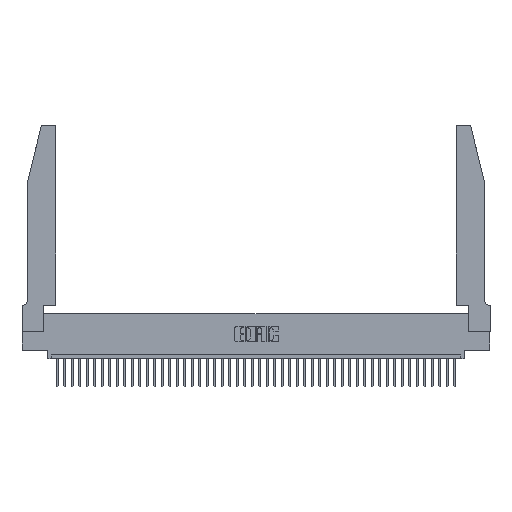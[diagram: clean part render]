
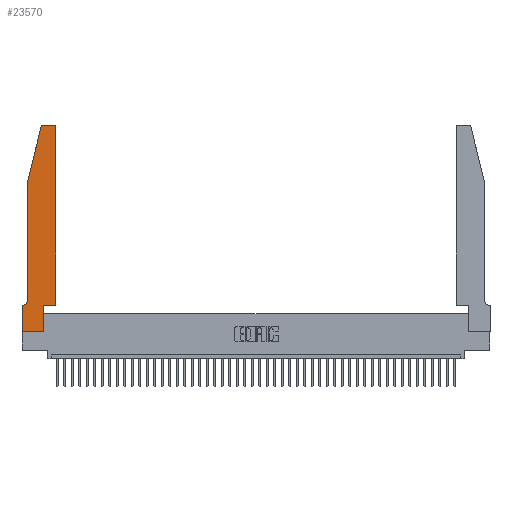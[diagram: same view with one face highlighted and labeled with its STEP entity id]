
A CAD part, top view. The second image highlights one B-rep face of the part: STEP entity #23570.
In plain terms, the highlighted planar face has unit normal (0, 0, 1).
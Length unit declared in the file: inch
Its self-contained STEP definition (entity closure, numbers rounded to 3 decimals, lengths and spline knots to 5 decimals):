
#668 = AXIS2_PLACEMENT_3D ( 'NONE', #10846, #24647, #20948 ) ;
#816 = CARTESIAN_POINT ( 'NONE',  ( 0.0755, 2., 0.37 ) ) ;
#941 = DIRECTION ( 'NONE',  ( -1., 0., 0. ) ) ;
#1044 = CIRCLE ( 'NONE', #10132, 0.03 ) ;
#1135 = CARTESIAN_POINT ( 'NONE',  ( 0.2865, 0.35, 0.37 ) ) ;
#1414 = VERTEX_POINT ( 'NONE', #2004 ) ;
#2004 = CARTESIAN_POINT ( 'NONE',  ( 0.4505, 0.35, 0.37 ) ) ;
#2997 = EDGE_CURVE ( 'NONE', #4055, #8257, #1044, .T. ) ;
#4055 = VERTEX_POINT ( 'NONE', #32065 ) ;
#4761 = ORIENTED_EDGE ( 'NONE', *, *, #34002, .T. ) ;
#5108 = EDGE_CURVE ( 'NONE', #13053, #29665, #31711, .T. ) ;
#5269 = DIRECTION ( 'NONE',  ( 0., 1., 0. ) ) ;
#5386 = EDGE_CURVE ( 'NONE', #9681, #40438, #21077, .T. ) ;
#5597 = DIRECTION ( 'NONE',  ( 1., 0., 0. ) ) ;
#7216 = ORIENTED_EDGE ( 'NONE', *, *, #5108, .T. ) ;
#7484 = CARTESIAN_POINT ( 'NONE',  ( 0., 0., 0.37 ) ) ;
#8257 = VERTEX_POINT ( 'NONE', #11931 ) ;
#8695 = CARTESIAN_POINT ( 'NONE',  ( 0., 0., 0.37 ) ) ;
#9653 = DIRECTION ( 'NONE',  ( 1., 0., 0. ) ) ;
#9681 = VERTEX_POINT ( 'NONE', #16517 ) ;
#10132 = AXIS2_PLACEMENT_3D ( 'NONE', #18822, #42362, #22064 ) ;
#10153 = DIRECTION ( 'NONE',  ( -0.239, -0.971, 0. ) ) ;
#10846 = CARTESIAN_POINT ( 'NONE',  ( 0.284, 2.72, 0.37 ) ) ;
#11004 = LINE ( 'NONE', #19722, #29632 ) ;
#11197 = CARTESIAN_POINT ( 'NONE',  ( 0.0755, 0.35, 0.37 ) ) ;
#11525 = VECTOR ( 'NONE', #5269, 39.37008 ) ;
#11547 = CARTESIAN_POINT ( 'NONE',  ( 0., 0.35, 0.37 ) ) ;
#11931 = CARTESIAN_POINT ( 'NONE',  ( 0.4205, 2.75, 0.37 ) ) ;
#12496 = VECTOR ( 'NONE', #18956, 39.37008 ) ;
#13053 = VERTEX_POINT ( 'NONE', #22299 ) ;
#13202 = VECTOR ( 'NONE', #10153, 39.37008 ) ;
#13825 = CARTESIAN_POINT ( 'NONE',  ( 0.0755, 0.42, 0.37 ) ) ;
#14412 = VECTOR ( 'NONE', #5597, 39.37008 ) ;
#14427 = VERTEX_POINT ( 'NONE', #13825 ) ;
#15261 = CARTESIAN_POINT ( 'NONE',  ( 0.0755, 2., 0.37 ) ) ;
#15931 = VECTOR ( 'NONE', #38326, 39.37008 ) ;
#16517 = CARTESIAN_POINT ( 'NONE',  ( 0.2865, 0., 0.37 ) ) ;
#18342 = ORIENTED_EDGE ( 'NONE', *, *, #22593, .T. ) ;
#18578 = LINE ( 'NONE', #33830, #21210 ) ;
#18591 = CARTESIAN_POINT ( 'NONE',  ( 0., 0.35, 0.37 ) ) ;
#18822 = CARTESIAN_POINT ( 'NONE',  ( 0.4205, 2.72, 0.37 ) ) ;
#18956 = DIRECTION ( 'NONE',  ( -1., 0., 0. ) ) ;
#19722 = CARTESIAN_POINT ( 'NONE',  ( 0.4505, 0.35, 0.37 ) ) ;
#19889 = EDGE_LOOP ( 'NONE', ( #4761, #30393, #7216, #40373, #22194, #21090, #22192, #24169, #32950, #18342, #26934, #23858 ) ) ;
#20124 = FACE_OUTER_BOUND ( 'NONE', #19889, .T. ) ;
#20133 = VERTEX_POINT ( 'NONE', #21171 ) ;
#20267 = CARTESIAN_POINT ( 'NONE',  ( 0.0755, 2., 0.37 ) ) ;
#20818 = AXIS2_PLACEMENT_3D ( 'NONE', #11547, #24437, #38428 ) ;
#20943 = CARTESIAN_POINT ( 'NONE',  ( 0.284, 2.75, 0.37 ) ) ;
#20948 = DIRECTION ( 'NONE',  ( 1., 0., 0. ) ) ;
#21077 = LINE ( 'NONE', #31662, #11525 ) ;
#21090 = ORIENTED_EDGE ( 'NONE', *, *, #36607, .T. ) ;
#21168 = CARTESIAN_POINT ( 'NONE',  ( 0.0055, 0.42, 0.37 ) ) ;
#21171 = CARTESIAN_POINT ( 'NONE',  ( 0., 0., 0.37 ) ) ;
#21177 = EDGE_CURVE ( 'NONE', #20133, #9681, #29898, .T. ) ;
#21210 = VECTOR ( 'NONE', #9653, 39.37008 ) ;
#21493 = LINE ( 'NONE', #42050, #12496 ) ;
#21993 = VECTOR ( 'NONE', #34496, 39.37008 ) ;
#22064 = DIRECTION ( 'NONE',  ( 1., 0., 0. ) ) ;
#22192 = ORIENTED_EDGE ( 'NONE', *, *, #25348, .T. ) ;
#22194 = ORIENTED_EDGE ( 'NONE', *, *, #41020, .T. ) ;
#22299 = CARTESIAN_POINT ( 'NONE',  ( 0.25487, 2.72718, 0.37 ) ) ;
#22593 = EDGE_CURVE ( 'NONE', #40438, #1414, #18578, .T. ) ;
#23095 = LINE ( 'NONE', #7484, #21993 ) ;
#23570 = ADVANCED_FACE ( 'NONE', ( #20124 ), #31889, .T. ) ;
#23644 = VERTEX_POINT ( 'NONE', #18591 ) ;
#23858 = ORIENTED_EDGE ( 'NONE', *, *, #2997, .T. ) ;
#24169 = ORIENTED_EDGE ( 'NONE', *, *, #21177, .T. ) ;
#24437 = DIRECTION ( 'NONE',  ( 0., 0., 1. ) ) ;
#24647 = DIRECTION ( 'NONE',  ( 0., 0., 1. ) ) ;
#25093 = CARTESIAN_POINT ( 'NONE',  ( 0.0055, 0.35, 0.37 ) ) ;
#25348 = EDGE_CURVE ( 'NONE', #23644, #20133, #23095, .T. ) ;
#25965 = CIRCLE ( 'NONE', #668, 0.03 ) ;
#26060 = VERTEX_POINT ( 'NONE', #25093 ) ;
#26934 = ORIENTED_EDGE ( 'NONE', *, *, #38062, .T. ) ;
#27208 = VERTEX_POINT ( 'NONE', #20943 ) ;
#27516 = EDGE_CURVE ( 'NONE', #29665, #14427, #43749, .T. ) ;
#28580 = AXIS2_PLACEMENT_3D ( 'NONE', #21168, #31984, #941 ) ;
#29632 = VECTOR ( 'NONE', #39733, 39.37008 ) ;
#29665 = VERTEX_POINT ( 'NONE', #816 ) ;
#29898 = LINE ( 'NONE', #8695, #14412 ) ;
#30393 = ORIENTED_EDGE ( 'NONE', *, *, #30825, .T. ) ;
#30825 = EDGE_CURVE ( 'NONE', #27208, #13053, #25965, .T. ) ;
#31662 = CARTESIAN_POINT ( 'NONE',  ( 0.2865, 0.35, 0.37 ) ) ;
#31711 = LINE ( 'NONE', #20267, #13202 ) ;
#31889 = PLANE ( 'NONE',  #20818 ) ;
#31984 = DIRECTION ( 'NONE',  ( 0., 0., -1. ) ) ;
#32065 = CARTESIAN_POINT ( 'NONE',  ( 0.4505, 2.72, 0.37 ) ) ;
#32088 = VECTOR ( 'NONE', #39476, 39.37008 ) ;
#32404 = LINE ( 'NONE', #11197, #15931 ) ;
#32950 = ORIENTED_EDGE ( 'NONE', *, *, #5386, .T. ) ;
#33830 = CARTESIAN_POINT ( 'NONE',  ( 0.4505, 0.35, 0.37 ) ) ;
#34002 = EDGE_CURVE ( 'NONE', #8257, #27208, #21493, .T. ) ;
#34496 = DIRECTION ( 'NONE',  ( 0., -1., 0. ) ) ;
#36607 = EDGE_CURVE ( 'NONE', #26060, #23644, #32404, .T. ) ;
#38062 = EDGE_CURVE ( 'NONE', #1414, #4055, #11004, .T. ) ;
#38326 = DIRECTION ( 'NONE',  ( -1., 0., 0. ) ) ;
#38428 = DIRECTION ( 'NONE',  ( 1., 0., 0. ) ) ;
#39476 = DIRECTION ( 'NONE',  ( 0., -1., 0. ) ) ;
#39733 = DIRECTION ( 'NONE',  ( 0., 1., 0. ) ) ;
#40373 = ORIENTED_EDGE ( 'NONE', *, *, #27516, .T. ) ;
#40438 = VERTEX_POINT ( 'NONE', #1135 ) ;
#41020 = EDGE_CURVE ( 'NONE', #14427, #26060, #42226, .T. ) ;
#42050 = CARTESIAN_POINT ( 'NONE',  ( 0.2605, 2.75, 0.37 ) ) ;
#42226 = CIRCLE ( 'NONE', #28580, 0.07 ) ;
#42362 = DIRECTION ( 'NONE',  ( 0., 0., 1. ) ) ;
#43749 = LINE ( 'NONE', #15261, #32088 ) ;
